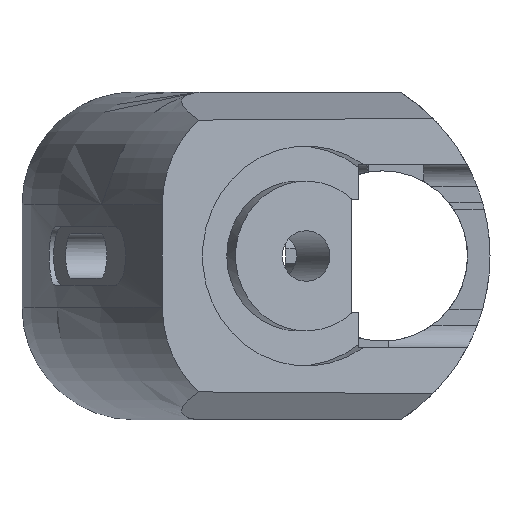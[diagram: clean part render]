
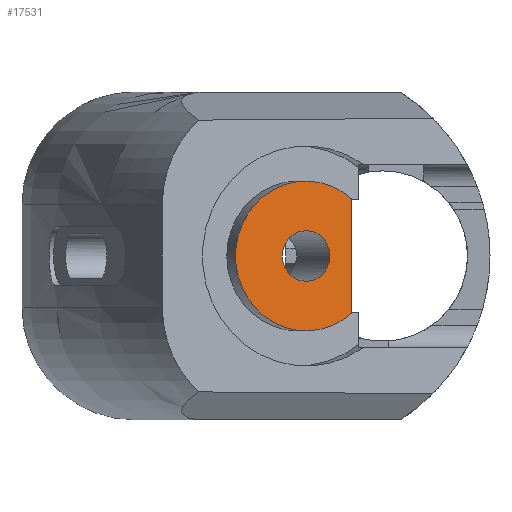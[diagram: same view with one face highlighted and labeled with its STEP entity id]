
A CAD part, left-side view. The second image highlights one B-rep face of the part: STEP entity #17531.
In plain terms, the highlighted planar face has unit normal (-0.943, -0.334, 0).
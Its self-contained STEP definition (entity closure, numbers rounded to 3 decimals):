
#3280 = PLANE('',#3281);
#3281 = AXIS2_PLACEMENT_3D('',#3282,#3283,#3284);
#3282 = CARTESIAN_POINT('',(-152.4,18.796,7.62));
#3283 = DIRECTION('',(0.,-1.,0.));
#3284 = DIRECTION('',(0.,0.,-1.));
#3329 = CYLINDRICAL_SURFACE('',#3330,3.429);
#3330 = AXIS2_PLACEMENT_3D('',#3331,#3332,#3333);
#3331 = CARTESIAN_POINT('',(-202.64,24.947,
    0.));
#3332 = DIRECTION('',(-0.943,-0.334,0.
    ));
#3333 = DIRECTION('',(0.334,-0.943,0.
    ));
#9529 = CYLINDRICAL_SURFACE('',#9530,10.16);
#9530 = AXIS2_PLACEMENT_3D('',#9531,#9532,#9533);
#9531 = CARTESIAN_POINT('',(-202.64,24.947,
    0.));
#9532 = DIRECTION('',(-0.943,-0.334,0.
    ));
#9533 = DIRECTION('',(0.334,-0.943,0.)
  );
#9717 = VERTEX_POINT('',#9718);
#9718 = CARTESIAN_POINT('',(-200.461,18.796,7.62));
#9732 = PLANE('',#9733);
#9733 = AXIS2_PLACEMENT_3D('',#9734,#9735,#9736);
#9734 = CARTESIAN_POINT('',(-152.4,17.78,7.62));
#9735 = DIRECTION('',(0.,0.,-1.));
#9736 = DIRECTION('',(0.,1.,0.));
#9744 = EDGE_CURVE('',#9717,#9745,#9747,.T.);
#9745 = VERTEX_POINT('',#9746);
#9746 = CARTESIAN_POINT('',(-200.461,18.796,-7.62));
#9747 = SURFACE_CURVE('',#9748,(#9752,#9758),.PCURVE_S1.);
#9748 = LINE('',#9749,#9750);
#9749 = CARTESIAN_POINT('',(-200.461,18.796,-7.303));
#9750 = VECTOR('',#9751,1.);
#9751 = DIRECTION('',(0.,0.,-1.));
#9752 = PCURVE('',#3280,#9753);
#9753 = DEFINITIONAL_REPRESENTATION('',(#9754),#9757);
#9754 = B_SPLINE_CURVE_WITH_KNOTS('',1,(#9755,#9756),.UNSPECIFIED.,.F.,
  .F.,(2,2),(-14.923,0.318),.PIECEWISE_BEZIER_KNOTS.);
#9755 = CARTESIAN_POINT('',(0.,-48.061));
#9756 = CARTESIAN_POINT('',(15.24,-48.061));
#9757 = ( GEOMETRIC_REPRESENTATION_CONTEXT(2) 
PARAMETRIC_REPRESENTATION_CONTEXT() REPRESENTATION_CONTEXT('2D SPACE',''
  ) );
#9758 = PCURVE('',#9759,#9764);
#9759 = PLANE('',#9760);
#9760 = AXIS2_PLACEMENT_3D('',#9761,#9762,#9763);
#9761 = CARTESIAN_POINT('',(-209.55,44.45,-22.225));
#9762 = DIRECTION('',(0.943,0.334,0.)
  );
#9763 = DIRECTION('',(0.334,-0.943,0.)
  );
#9764 = DEFINITIONAL_REPRESENTATION('',(#9765),#9768);
#9765 = B_SPLINE_CURVE_WITH_KNOTS('',1,(#9766,#9767),.UNSPECIFIED.,.F.,
  .F.,(2,2),(-14.923,0.318),.PIECEWISE_BEZIER_KNOTS.);
#9766 = CARTESIAN_POINT('',(27.216,-29.845));
#9767 = CARTESIAN_POINT('',(27.216,-14.605));
#9768 = ( GEOMETRIC_REPRESENTATION_CONTEXT(2) 
PARAMETRIC_REPRESENTATION_CONTEXT() REPRESENTATION_CONTEXT('2D SPACE',''
  ) );
#9786 = PLANE('',#9787);
#9787 = AXIS2_PLACEMENT_3D('',#9788,#9789,#9790);
#9788 = CARTESIAN_POINT('',(-152.4,18.796,-7.62));
#9789 = DIRECTION('',(0.,0.,1.));
#9790 = DIRECTION('',(0.,-1.,0.));
#9884 = EDGE_CURVE('',#9885,#9885,#9887,.T.);
#9885 = VERTEX_POINT('',#9886);
#9886 = CARTESIAN_POINT('',(-201.495,21.715,
    0.));
#9887 = SURFACE_CURVE('',#9888,(#9893,#9900),.PCURVE_S1.);
#9888 = CIRCLE('',#9889,3.429);
#9889 = AXIS2_PLACEMENT_3D('',#9890,#9891,#9892);
#9890 = CARTESIAN_POINT('',(-202.64,24.947,
    0.));
#9891 = DIRECTION('',(-0.943,-0.334,0.
    ));
#9892 = DIRECTION('',(0.334,-0.943,0.
    ));
#9893 = PCURVE('',#3329,#9894);
#9894 = DEFINITIONAL_REPRESENTATION('',(#9895),#9899);
#9895 = LINE('',#9896,#9897);
#9896 = CARTESIAN_POINT('',(0.,0.));
#9897 = VECTOR('',#9898,1.);
#9898 = DIRECTION('',(1.,0.));
#9899 = ( GEOMETRIC_REPRESENTATION_CONTEXT(2) 
PARAMETRIC_REPRESENTATION_CONTEXT() REPRESENTATION_CONTEXT('2D SPACE',''
  ) );
#9900 = PCURVE('',#9759,#9901);
#9901 = DEFINITIONAL_REPRESENTATION('',(#9902),#9910);
#9902 = ( BOUNDED_CURVE() B_SPLINE_CURVE(2,(#9903,#9904,#9905,#9906,
#9907,#9908,#9909),.UNSPECIFIED.,.T.,.F.) B_SPLINE_CURVE_WITH_KNOTS((1,2
    ,2,2,2,1),(-2.094,0.,2.094,4.189,
6.283,8.378),.UNSPECIFIED.) CURVE() 
GEOMETRIC_REPRESENTATION_ITEM() RATIONAL_B_SPLINE_CURVE((1.,0.5,1.,0.5,
1.,0.5,1.)) REPRESENTATION_ITEM('') );
#9903 = CARTESIAN_POINT('',(24.12,-22.225));
#9904 = CARTESIAN_POINT('',(24.12,-28.164));
#9905 = CARTESIAN_POINT('',(18.976,-25.195));
#9906 = CARTESIAN_POINT('',(13.833,-22.225));
#9907 = CARTESIAN_POINT('',(18.976,-19.255));
#9908 = CARTESIAN_POINT('',(24.12,-16.286));
#9909 = CARTESIAN_POINT('',(24.12,-22.225));
#9910 = ( GEOMETRIC_REPRESENTATION_CONTEXT(2) 
PARAMETRIC_REPRESENTATION_CONTEXT() REPRESENTATION_CONTEXT('2D SPACE',''
  ) );
#17155 = EDGE_CURVE('',#17156,#17158,#17160,.T.);
#17156 = VERTEX_POINT('',#17157);
#17157 = CARTESIAN_POINT('',(-200.396,18.613,7.62));
#17158 = VERTEX_POINT('',#17159);
#17159 = CARTESIAN_POINT('',(-200.396,18.613,-7.62));
#17160 = SURFACE_CURVE('',#17161,(#17166,#17173),.PCURVE_S1.);
#17161 = CIRCLE('',#17162,10.16);
#17162 = AXIS2_PLACEMENT_3D('',#17163,#17164,#17165);
#17163 = CARTESIAN_POINT('',(-202.64,24.947,
    0.));
#17164 = DIRECTION('',(-0.943,-0.334,
    0.));
#17165 = DIRECTION('',(0.334,-0.943,0.
    ));
#17166 = PCURVE('',#9529,#17167);
#17167 = DEFINITIONAL_REPRESENTATION('',(#17168),#17172);
#17168 = LINE('',#17169,#17170);
#17169 = CARTESIAN_POINT('',(0.,0.));
#17170 = VECTOR('',#17171,1.);
#17171 = DIRECTION('',(1.,0.));
#17172 = ( GEOMETRIC_REPRESENTATION_CONTEXT(2) 
PARAMETRIC_REPRESENTATION_CONTEXT() REPRESENTATION_CONTEXT('2D SPACE',''
  ) );
#17173 = PCURVE('',#9759,#17174);
#17174 = DEFINITIONAL_REPRESENTATION('',(#17175),#17183);
#17175 = ( BOUNDED_CURVE() B_SPLINE_CURVE(2,(#17176,#17177,#17178,#17179
    ,#17180,#17181,#17182),.UNSPECIFIED.,.T.,.F.) 
B_SPLINE_CURVE_WITH_KNOTS((1,2,2,2,2,1),(-2.094,0.,
    2.094,4.189,6.283,8.378),
.UNSPECIFIED.) CURVE() GEOMETRIC_REPRESENTATION_ITEM() 
RATIONAL_B_SPLINE_CURVE((1.,0.5,1.,0.5,1.,0.5,1.)) REPRESENTATION_ITEM(
  '') );
#17176 = CARTESIAN_POINT('',(30.851,-22.225));
#17177 = CARTESIAN_POINT('',(30.851,-39.823));
#17178 = CARTESIAN_POINT('',(15.611,-31.024));
#17179 = CARTESIAN_POINT('',(0.371,-22.225));
#17180 = CARTESIAN_POINT('',(15.611,-13.426));
#17181 = CARTESIAN_POINT('',(30.851,-4.627));
#17182 = CARTESIAN_POINT('',(30.851,-22.225));
#17183 = ( GEOMETRIC_REPRESENTATION_CONTEXT(2) 
PARAMETRIC_REPRESENTATION_CONTEXT() REPRESENTATION_CONTEXT('2D SPACE',''
  ) );
#17513 = EDGE_CURVE('',#9745,#17158,#17514,.T.);
#17514 = SURFACE_CURVE('',#17515,(#17519,#17525),.PCURVE_S1.);
#17515 = LINE('',#17516,#17517);
#17516 = CARTESIAN_POINT('',(-202.326,24.059,-7.62));
#17517 = VECTOR('',#17518,1.);
#17518 = DIRECTION('',(0.334,-0.943,0.
    ));
#17519 = PCURVE('',#9786,#17520);
#17520 = DEFINITIONAL_REPRESENTATION('',(#17521),#17524);
#17521 = B_SPLINE_CURVE_WITH_KNOTS('',1,(#17522,#17523),.UNSPECIFIED.,
  .F.,.F.,(2,2),(5.583,6.661),
  .PIECEWISE_BEZIER_KNOTS.);
#17522 = CARTESIAN_POINT('',(0.,-48.061));
#17523 = CARTESIAN_POINT('',(1.016,-47.701));
#17524 = ( GEOMETRIC_REPRESENTATION_CONTEXT(2) 
PARAMETRIC_REPRESENTATION_CONTEXT() REPRESENTATION_CONTEXT('2D SPACE',''
  ) );
#17525 = PCURVE('',#9759,#17526);
#17526 = DEFINITIONAL_REPRESENTATION('',(#17527),#17530);
#17527 = B_SPLINE_CURVE_WITH_KNOTS('',1,(#17528,#17529),.UNSPECIFIED.,
  .F.,.F.,(2,2),(5.583,6.661),
  .PIECEWISE_BEZIER_KNOTS.);
#17528 = CARTESIAN_POINT('',(27.216,-14.605));
#17529 = CARTESIAN_POINT('',(28.294,-14.605));
#17530 = ( GEOMETRIC_REPRESENTATION_CONTEXT(2) 
PARAMETRIC_REPRESENTATION_CONTEXT() REPRESENTATION_CONTEXT('2D SPACE',''
  ) );
#17531 = ADVANCED_FACE('',(#17532,#17556),#9759,.F.);
#17532 = FACE_BOUND('',#17533,.F.);
#17533 = EDGE_LOOP('',(#17534,#17535,#17536,#17555));
#17534 = ORIENTED_EDGE('',*,*,#17513,.T.);
#17535 = ORIENTED_EDGE('',*,*,#17155,.F.);
#17536 = ORIENTED_EDGE('',*,*,#17537,.T.);
#17537 = EDGE_CURVE('',#17156,#9717,#17538,.T.);
#17538 = SURFACE_CURVE('',#17539,(#17543,#17549),.PCURVE_S1.);
#17539 = LINE('',#17540,#17541);
#17540 = CARTESIAN_POINT('',(-202.166,23.607,7.62));
#17541 = VECTOR('',#17542,1.);
#17542 = DIRECTION('',(-0.334,0.943,
    0.));
#17543 = PCURVE('',#9759,#17544);
#17544 = DEFINITIONAL_REPRESENTATION('',(#17545),#17548);
#17545 = B_SPLINE_CURVE_WITH_KNOTS('',1,(#17546,#17547),.UNSPECIFIED.,
  .F.,.F.,(2,2),(-6.182,-5.104),
  .PIECEWISE_BEZIER_KNOTS.);
#17546 = CARTESIAN_POINT('',(28.294,-29.845));
#17547 = CARTESIAN_POINT('',(27.216,-29.845));
#17548 = ( GEOMETRIC_REPRESENTATION_CONTEXT(2) 
PARAMETRIC_REPRESENTATION_CONTEXT() REPRESENTATION_CONTEXT('2D SPACE',''
  ) );
#17549 = PCURVE('',#9732,#17550);
#17550 = DEFINITIONAL_REPRESENTATION('',(#17551),#17554);
#17551 = B_SPLINE_CURVE_WITH_KNOTS('',1,(#17552,#17553),.UNSPECIFIED.,
  .F.,.F.,(2,2),(-6.182,-5.104),
  .PIECEWISE_BEZIER_KNOTS.);
#17552 = CARTESIAN_POINT('',(0.,-47.701));
#17553 = CARTESIAN_POINT('',(1.016,-48.061));
#17554 = ( GEOMETRIC_REPRESENTATION_CONTEXT(2) 
PARAMETRIC_REPRESENTATION_CONTEXT() REPRESENTATION_CONTEXT('2D SPACE',''
  ) );
#17555 = ORIENTED_EDGE('',*,*,#9744,.T.);
#17556 = FACE_BOUND('',#17557,.F.);
#17557 = EDGE_LOOP('',(#17558));
#17558 = ORIENTED_EDGE('',*,*,#9884,.T.);
